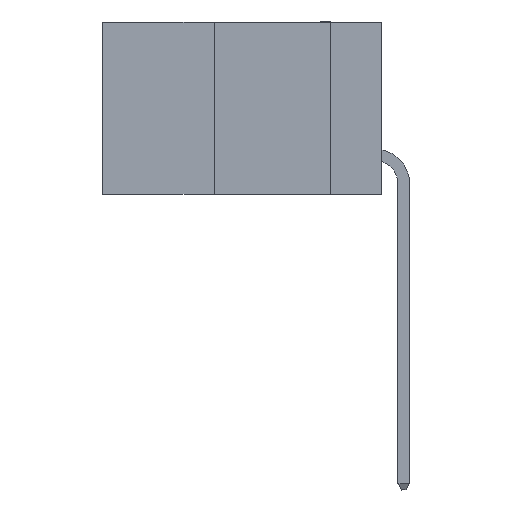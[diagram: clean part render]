
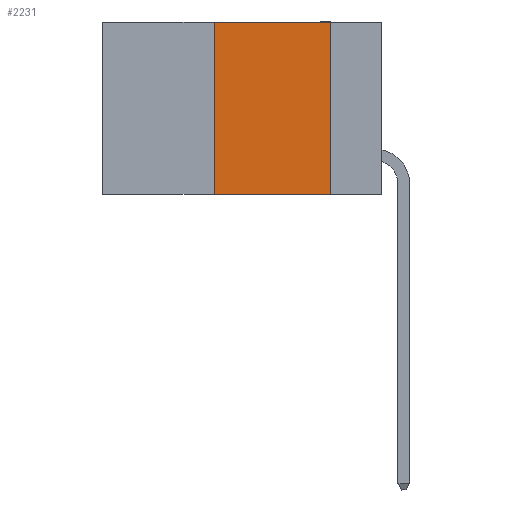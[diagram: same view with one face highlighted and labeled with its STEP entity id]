
A CAD part, left-side view. The second image highlights one B-rep face of the part: STEP entity #2231.
In plain terms, the highlighted planar face has unit normal (-1, 0, 0).
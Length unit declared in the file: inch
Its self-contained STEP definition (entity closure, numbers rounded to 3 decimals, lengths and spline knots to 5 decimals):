
#447 = LINE ( 'NONE', #24024, #824 ) ;
#753 = VERTEX_POINT ( 'NONE', #7846 ) ;
#824 = VECTOR ( 'NONE', #21885, 39.37008 ) ;
#1060 = EDGE_CURVE ( 'NONE', #753, #1343, #14755, .T. ) ;
#1320 = CARTESIAN_POINT ( 'NONE',  ( 0., 0.6, 0. ) ) ;
#1343 = VERTEX_POINT ( 'NONE', #29190 ) ;
#1584 = CARTESIAN_POINT ( 'NONE',  ( 0., 0.11, -0.37 ) ) ;
#1701 = ORIENTED_EDGE ( 'NONE', *, *, #4784, .F. ) ;
#2231 = ADVANCED_FACE ( 'NONE', ( #21175 ), #11336, .F. ) ;
#3489 = EDGE_CURVE ( 'NONE', #1343, #3778, #25809, .T. ) ;
#3778 = VERTEX_POINT ( 'NONE', #1584 ) ;
#4105 = CARTESIAN_POINT ( 'NONE',  ( 0., 0.36, -0.37 ) ) ;
#4784 = EDGE_CURVE ( 'NONE', #28836, #753, #447, .T. ) ;
#4964 = ORIENTED_EDGE ( 'NONE', *, *, #21068, .T. ) ;
#7014 = VECTOR ( 'NONE', #11952, 39.37008 ) ;
#7846 = CARTESIAN_POINT ( 'NONE',  ( 0., 0.36, 0. ) ) ;
#7870 = VECTOR ( 'NONE', #23791, 39.37008 ) ;
#11336 = PLANE ( 'NONE',  #16516 ) ;
#11952 = DIRECTION ( 'NONE',  ( 0., 0., -1. ) ) ;
#12706 = ORIENTED_EDGE ( 'NONE', *, *, #1060, .F. ) ;
#14386 = CARTESIAN_POINT ( 'NONE',  ( 0., 0.6, 0. ) ) ;
#14755 = LINE ( 'NONE', #14386, #7870 ) ;
#16516 = AXIS2_PLACEMENT_3D ( 'NONE', #1320, #22083, #17611 ) ;
#17611 = DIRECTION ( 'NONE',  ( 0., 0., -1. ) ) ;
#17874 = DIRECTION ( 'NONE',  ( 0., -1., 0. ) ) ;
#18839 = LINE ( 'NONE', #29297, #26817 ) ;
#21043 = EDGE_LOOP ( 'NONE', ( #27500, #12706, #1701, #4964 ) ) ;
#21068 = EDGE_CURVE ( 'NONE', #28836, #3778, #18839, .T. ) ;
#21175 = FACE_OUTER_BOUND ( 'NONE', #21043, .T. ) ;
#21793 = CARTESIAN_POINT ( 'NONE',  ( 0., 0.11, 0. ) ) ;
#21885 = DIRECTION ( 'NONE',  ( 0., 0., 1. ) ) ;
#22083 = DIRECTION ( 'NONE',  ( 1., 0., 0. ) ) ;
#23791 = DIRECTION ( 'NONE',  ( 0., -1., 0. ) ) ;
#24024 = CARTESIAN_POINT ( 'NONE',  ( 0., 0.36, 0. ) ) ;
#25809 = LINE ( 'NONE', #21793, #7014 ) ;
#26817 = VECTOR ( 'NONE', #17874, 39.37008 ) ;
#27500 = ORIENTED_EDGE ( 'NONE', *, *, #3489, .F. ) ;
#28836 = VERTEX_POINT ( 'NONE', #4105 ) ;
#29190 = CARTESIAN_POINT ( 'NONE',  ( 0., 0.11, 0. ) ) ;
#29297 = CARTESIAN_POINT ( 'NONE',  ( 0., 0.6, -0.37 ) ) ;
